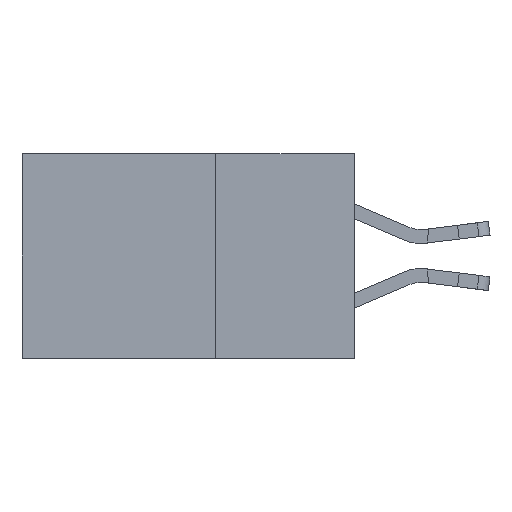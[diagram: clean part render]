
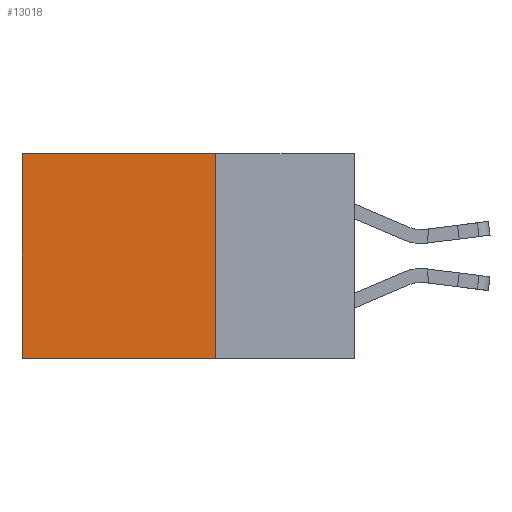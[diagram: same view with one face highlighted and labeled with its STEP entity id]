
A CAD part, left-side view. The second image highlights one B-rep face of the part: STEP entity #13018.
In plain terms, the highlighted planar face has unit normal (-1, 0, 0).
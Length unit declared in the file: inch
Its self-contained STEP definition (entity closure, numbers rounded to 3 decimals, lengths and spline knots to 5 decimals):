
#121 = AXIS2_PLACEMENT_3D ( 'NONE', #10095, #5516, #13644 ) ;
#318 = EDGE_CURVE ( 'NONE', #14104, #13590, #3514, .T. ) ;
#594 = CARTESIAN_POINT ( 'NONE',  ( 0.298, 0.6, 0. ) ) ;
#842 = VECTOR ( 'NONE', #1162, 39.37008 ) ;
#1162 = DIRECTION ( 'NONE',  ( 0., 0., -1. ) ) ;
#1967 = ORIENTED_EDGE ( 'NONE', *, *, #8905, .F. ) ;
#2642 = LINE ( 'NONE', #5393, #11763 ) ;
#3183 = CARTESIAN_POINT ( 'NONE',  ( 0.298, 0.6, 0. ) ) ;
#3514 = LINE ( 'NONE', #3183, #842 ) ;
#3897 = LINE ( 'NONE', #10699, #9646 ) ;
#4014 = EDGE_CURVE ( 'NONE', #5508, #14104, #2642, .T. ) ;
#4221 = ORIENTED_EDGE ( 'NONE', *, *, #318, .T. ) ;
#4839 = DIRECTION ( 'NONE',  ( 0., 1., 0. ) ) ;
#5249 = ORIENTED_EDGE ( 'NONE', *, *, #4014, .T. ) ;
#5393 = CARTESIAN_POINT ( 'NONE',  ( 0.298, 0.25, 0. ) ) ;
#5508 = VERTEX_POINT ( 'NONE', #8685 ) ;
#5516 = DIRECTION ( 'NONE',  ( 1., 0., 0. ) ) ;
#5880 = CARTESIAN_POINT ( 'NONE',  ( 0.298, 0.25, 0. ) ) ;
#6395 = LINE ( 'NONE', #5880, #10265 ) ;
#7659 = CARTESIAN_POINT ( 'NONE',  ( 0.298, 0.6, -0.37 ) ) ;
#8101 = VERTEX_POINT ( 'NONE', #12716 ) ;
#8685 = CARTESIAN_POINT ( 'NONE',  ( 0.298, 0.25, 0. ) ) ;
#8905 = EDGE_CURVE ( 'NONE', #5508, #8101, #6395, .T. ) ;
#9646 = VECTOR ( 'NONE', #11849, 39.37008 ) ;
#9963 = FACE_OUTER_BOUND ( 'NONE', #12260, .T. ) ;
#10095 = CARTESIAN_POINT ( 'NONE',  ( 0.298, 0.25, 0. ) ) ;
#10265 = VECTOR ( 'NONE', #14004, 39.37008 ) ;
#10699 = CARTESIAN_POINT ( 'NONE',  ( 0.298, 0.25, -0.37 ) ) ;
#11763 = VECTOR ( 'NONE', #4839, 39.37008 ) ;
#11849 = DIRECTION ( 'NONE',  ( 0., 1., 0. ) ) ;
#12108 = EDGE_CURVE ( 'NONE', #8101, #13590, #3897, .T. ) ;
#12260 = EDGE_LOOP ( 'NONE', ( #4221, #13791, #1967, #5249 ) ) ;
#12515 = PLANE ( 'NONE',  #121 ) ;
#12716 = CARTESIAN_POINT ( 'NONE',  ( 0.298, 0.25, -0.37 ) ) ;
#13018 = ADVANCED_FACE ( 'NONE', ( #9963 ), #12515, .F. ) ;
#13590 = VERTEX_POINT ( 'NONE', #7659 ) ;
#13644 = DIRECTION ( 'NONE',  ( 0., 0., -1. ) ) ;
#13791 = ORIENTED_EDGE ( 'NONE', *, *, #12108, .F. ) ;
#14004 = DIRECTION ( 'NONE',  ( 0., 0., -1. ) ) ;
#14104 = VERTEX_POINT ( 'NONE', #594 ) ;
